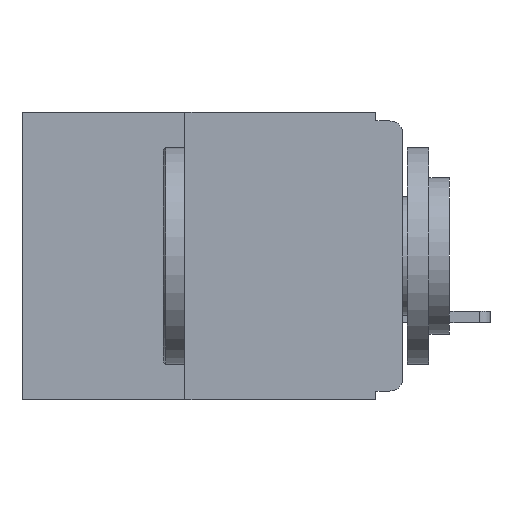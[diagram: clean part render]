
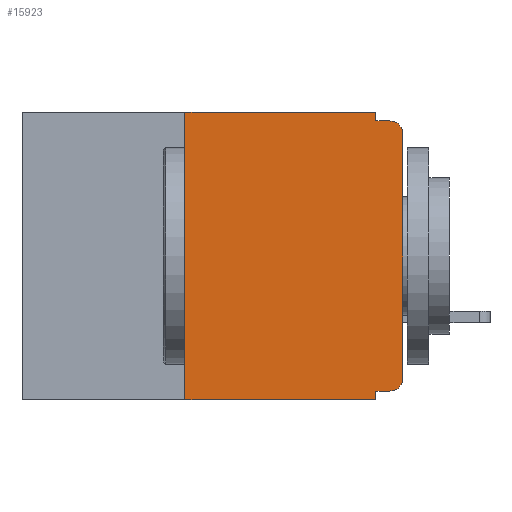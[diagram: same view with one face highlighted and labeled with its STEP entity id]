
A CAD part, left-side view. The second image highlights one B-rep face of the part: STEP entity #15923.
In plain terms, the highlighted planar face has unit normal (-1, 0, 0).
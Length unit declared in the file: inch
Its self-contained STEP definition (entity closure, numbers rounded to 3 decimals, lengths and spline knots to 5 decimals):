
#17 = CARTESIAN_POINT ( 'NONE',  ( 0., 0., 0. ) ) ;
#114 = CARTESIAN_POINT ( 'NONE',  ( 0., 0.25, -0.33 ) ) ;
#364 = DIRECTION ( 'NONE',  ( 0., 1., 0. ) ) ;
#529 = EDGE_CURVE ( 'NONE', #16204, #17825, #10354, .T. ) ;
#1021 = CARTESIAN_POINT ( 'NONE',  ( 0., 0.015, -0.01 ) ) ;
#1171 = VECTOR ( 'NONE', #16668, 39.37008 ) ;
#1437 = DIRECTION ( 'NONE',  ( 0., 0., -1. ) ) ;
#1480 = VECTOR ( 'NONE', #15262, 39.37008 ) ;
#1617 = CIRCLE ( 'NONE', #15246, 0.015 ) ;
#1656 = CARTESIAN_POINT ( 'NONE',  ( 0., 0.015, -0.025 ) ) ;
#1710 = DIRECTION ( 'NONE',  ( 0., 0., -1. ) ) ;
#1869 = DIRECTION ( 'NONE',  ( -1., 0., 0. ) ) ;
#2379 = EDGE_CURVE ( 'NONE', #19192, #2908, #16524, .T. ) ;
#2613 = CARTESIAN_POINT ( 'NONE',  ( 0., 0.015, -0.32 ) ) ;
#2766 = EDGE_CURVE ( 'NONE', #2908, #4339, #1617, .T. ) ;
#2908 = VERTEX_POINT ( 'NONE', #13559 ) ;
#3056 = VECTOR ( 'NONE', #18892, 39.37008 ) ;
#3203 = VERTEX_POINT ( 'NONE', #17120 ) ;
#3340 = ORIENTED_EDGE ( 'NONE', *, *, #18672, .F. ) ;
#3799 = ORIENTED_EDGE ( 'NONE', *, *, #5508, .T. ) ;
#4339 = VERTEX_POINT ( 'NONE', #1021 ) ;
#4950 = ORIENTED_EDGE ( 'NONE', *, *, #2766, .T. ) ;
#5410 = ORIENTED_EDGE ( 'NONE', *, *, #5453, .F. ) ;
#5453 = EDGE_CURVE ( 'NONE', #14181, #4339, #17772, .T. ) ;
#5483 = FACE_OUTER_BOUND ( 'NONE', #16021, .T. ) ;
#5508 = EDGE_CURVE ( 'NONE', #14045, #19192, #16857, .T. ) ;
#5858 = CARTESIAN_POINT ( 'NONE',  ( 0., 0.437, 0. ) ) ;
#5913 = VECTOR ( 'NONE', #14978, 39.37008 ) ;
#6127 = CARTESIAN_POINT ( 'NONE',  ( 0., 0.437, 0. ) ) ;
#6324 = ORIENTED_EDGE ( 'NONE', *, *, #529, .F. ) ;
#7474 = LINE ( 'NONE', #18147, #14936 ) ;
#7651 = CARTESIAN_POINT ( 'NONE',  ( 0., 0.031, 0. ) ) ;
#8359 = ORIENTED_EDGE ( 'NONE', *, *, #2379, .T. ) ;
#8658 = VECTOR ( 'NONE', #8938, 39.37008 ) ;
#8938 = DIRECTION ( 'NONE',  ( 0., 0., 1. ) ) ;
#9758 = DIRECTION ( 'NONE',  ( 0., -1., 0. ) ) ;
#10244 = ORIENTED_EDGE ( 'NONE', *, *, #15530, .F. ) ;
#10312 = DIRECTION ( 'NONE',  ( 1., 0., 0. ) ) ;
#10354 = LINE ( 'NONE', #6127, #13844 ) ;
#10912 = LINE ( 'NONE', #17440, #3056 ) ;
#10945 = DIRECTION ( 'NONE',  ( 0., -1., 0. ) ) ;
#11123 = VERTEX_POINT ( 'NONE', #12047 ) ;
#12047 = CARTESIAN_POINT ( 'NONE',  ( 0., 0.031, -0.32 ) ) ;
#12721 = CARTESIAN_POINT ( 'NONE',  ( 0., 0.437, -0.33 ) ) ;
#12847 = VECTOR ( 'NONE', #9758, 39.37008 ) ;
#13244 = ORIENTED_EDGE ( 'NONE', *, *, #16787, .F. ) ;
#13559 = CARTESIAN_POINT ( 'NONE',  ( 0., 0., -0.025 ) ) ;
#13732 = CARTESIAN_POINT ( 'NONE',  ( 0., 0.031, 0. ) ) ;
#13844 = VECTOR ( 'NONE', #10945, 39.37008 ) ;
#13890 = AXIS2_PLACEMENT_3D ( 'NONE', #5858, #10312, #1437 ) ;
#14045 = VERTEX_POINT ( 'NONE', #2613 ) ;
#14174 = DIRECTION ( 'NONE',  ( 0., 0., -1. ) ) ;
#14181 = VERTEX_POINT ( 'NONE', #14812 ) ;
#14193 = DIRECTION ( 'NONE',  ( -1., 0., 0. ) ) ;
#14238 = CARTESIAN_POINT ( 'NONE',  ( 0., 0.015, -0.305 ) ) ;
#14674 = ORIENTED_EDGE ( 'NONE', *, *, #15242, .T. ) ;
#14812 = CARTESIAN_POINT ( 'NONE',  ( 0., 0.031, -0.01 ) ) ;
#14936 = VECTOR ( 'NONE', #364, 39.37008 ) ;
#14978 = DIRECTION ( 'NONE',  ( 0., -1., 0. ) ) ;
#15019 = CARTESIAN_POINT ( 'NONE',  ( 0., 0., -0.01 ) ) ;
#15181 = VERTEX_POINT ( 'NONE', #15587 ) ;
#15242 = EDGE_CURVE ( 'NONE', #15181, #3203, #17327, .T. ) ;
#15246 = AXIS2_PLACEMENT_3D ( 'NONE', #1656, #1869, #1710 ) ;
#15262 = DIRECTION ( 'NONE',  ( 0., 0., -1. ) ) ;
#15413 = CARTESIAN_POINT ( 'NONE',  ( 0., 0.25, 0. ) ) ;
#15530 = EDGE_CURVE ( 'NONE', #15181, #16204, #16162, .T. ) ;
#15587 = CARTESIAN_POINT ( 'NONE',  ( 0., 0.25, -0.33 ) ) ;
#15923 = ADVANCED_FACE ( 'NONE', ( #5483 ), #19198, .F. ) ;
#16021 = EDGE_LOOP ( 'NONE', ( #8359, #4950, #5410, #13244, #6324, #10244, #14674, #3340, #19064, #3799 ) ) ;
#16162 = LINE ( 'NONE', #114, #8658 ) ;
#16204 = VERTEX_POINT ( 'NONE', #15413 ) ;
#16524 = LINE ( 'NONE', #17, #1171 ) ;
#16668 = DIRECTION ( 'NONE',  ( 0., 0., 1. ) ) ;
#16787 = EDGE_CURVE ( 'NONE', #17825, #14181, #17760, .T. ) ;
#16857 = CIRCLE ( 'NONE', #18488, 0.015 ) ;
#17120 = CARTESIAN_POINT ( 'NONE',  ( 0., 0.031, -0.33 ) ) ;
#17165 = CARTESIAN_POINT ( 'NONE',  ( 0., 0., -0.305 ) ) ;
#17327 = LINE ( 'NONE', #12721, #12847 ) ;
#17336 = EDGE_CURVE ( 'NONE', #14045, #11123, #7474, .T. ) ;
#17440 = CARTESIAN_POINT ( 'NONE',  ( 0., 0.031, -0.33 ) ) ;
#17760 = LINE ( 'NONE', #13732, #1480 ) ;
#17772 = LINE ( 'NONE', #15019, #5913 ) ;
#17825 = VERTEX_POINT ( 'NONE', #7651 ) ;
#18147 = CARTESIAN_POINT ( 'NONE',  ( 0., 0., -0.32 ) ) ;
#18488 = AXIS2_PLACEMENT_3D ( 'NONE', #14238, #14193, #14174 ) ;
#18672 = EDGE_CURVE ( 'NONE', #11123, #3203, #10912, .T. ) ;
#18892 = DIRECTION ( 'NONE',  ( 0., 0., -1. ) ) ;
#19064 = ORIENTED_EDGE ( 'NONE', *, *, #17336, .F. ) ;
#19192 = VERTEX_POINT ( 'NONE', #17165 ) ;
#19198 = PLANE ( 'NONE',  #13890 ) ;
